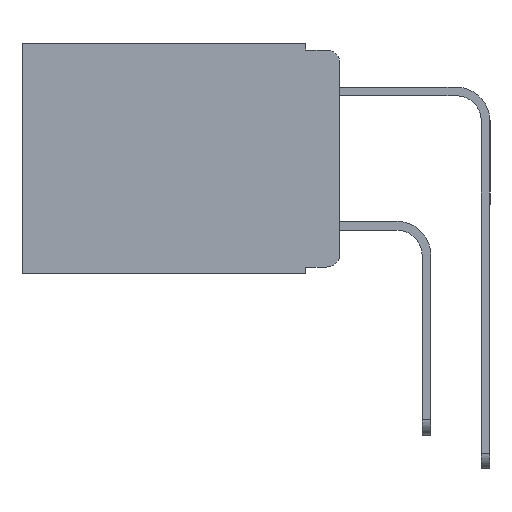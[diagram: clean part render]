
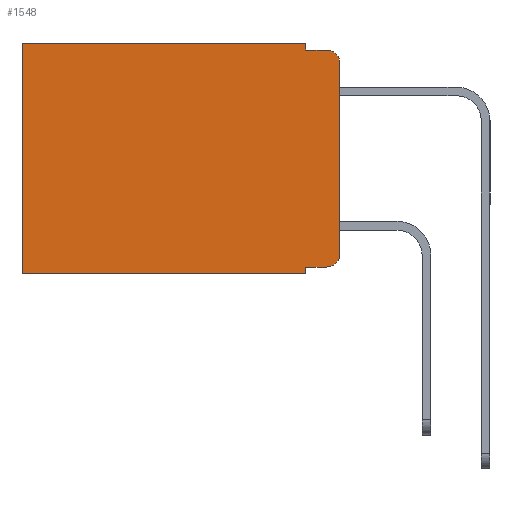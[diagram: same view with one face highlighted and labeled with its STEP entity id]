
A CAD part, left-side view. The second image highlights one B-rep face of the part: STEP entity #1548.
In plain terms, the highlighted planar face has unit normal (-1, 0, 0).
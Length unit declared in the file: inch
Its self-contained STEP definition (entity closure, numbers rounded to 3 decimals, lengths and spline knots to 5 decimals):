
#52 = VERTEX_POINT ( 'NONE', #1079 ) ;
#53 = CARTESIAN_POINT ( 'NONE',  ( 0.298, 0., 0. ) ) ;
#161 = CARTESIAN_POINT ( 'NONE',  ( 0.298, 0.473, 0. ) ) ;
#314 = DIRECTION ( 'NONE',  ( -1., 0., 0. ) ) ;
#1079 = CARTESIAN_POINT ( 'NONE',  ( 0.298, 0.051, -0.333 ) ) ;
#1282 = VECTOR ( 'NONE', #4727, 39.37008 ) ;
#1391 = VERTEX_POINT ( 'NONE', #13516 ) ;
#1548 = ADVANCED_FACE ( 'NONE', ( #12957 ), #14495, .F. ) ;
#1565 = CARTESIAN_POINT ( 'NONE',  ( 0.298, 0., 0. ) ) ;
#1922 = LINE ( 'NONE', #53, #8721 ) ;
#2081 = AXIS2_PLACEMENT_3D ( 'NONE', #3588, #12886, #4955 ) ;
#2167 = AXIS2_PLACEMENT_3D ( 'NONE', #8548, #314, #9907 ) ;
#2639 = EDGE_LOOP ( 'NONE', ( #9447, #10034, #13676, #13838, #10603, #10833, #13771, #11213, #11817, #11562 ) ) ;
#2655 = DIRECTION ( 'NONE',  ( 0., 1., 0. ) ) ;
#2825 = VECTOR ( 'NONE', #10303, 39.37008 ) ;
#3288 = LINE ( 'NONE', #8969, #2825 ) ;
#3350 = CARTESIAN_POINT ( 'NONE',  ( 0.298, 0.051, 0. ) ) ;
#3588 = CARTESIAN_POINT ( 'NONE',  ( 0.298, 0.02, -0.313 ) ) ;
#3645 = DIRECTION ( 'NONE',  ( 0., 0., -1. ) ) ;
#3745 = VECTOR ( 'NONE', #2655, 39.37008 ) ;
#4056 = CARTESIAN_POINT ( 'NONE',  ( 0.298, 0.473, -0.343 ) ) ;
#4166 = CIRCLE ( 'NONE', #2081, 0.02 ) ;
#4727 = DIRECTION ( 'NONE',  ( 0., 0., -1. ) ) ;
#4955 = DIRECTION ( 'NONE',  ( 0., 0., -1. ) ) ;
#5181 = VECTOR ( 'NONE', #7122, 39.37008 ) ;
#5445 = LINE ( 'NONE', #9951, #8520 ) ;
#6330 = CARTESIAN_POINT ( 'NONE',  ( 0.298, 0.051, -0.343 ) ) ;
#6504 = LINE ( 'NONE', #14199, #13085 ) ;
#6538 = CARTESIAN_POINT ( 'NONE',  ( 0.298, 0.051, -0.01 ) ) ;
#6722 = VERTEX_POINT ( 'NONE', #8576 ) ;
#6908 = LINE ( 'NONE', #16805, #13487 ) ;
#7121 = CIRCLE ( 'NONE', #2167, 0.02 ) ;
#7122 = DIRECTION ( 'NONE',  ( 0., 1., 0. ) ) ;
#7329 = LINE ( 'NONE', #10708, #3745 ) ;
#7433 = AXIS2_PLACEMENT_3D ( 'NONE', #1565, #11981, #8709 ) ;
#7658 = DIRECTION ( 'NONE',  ( 0., -1., 0. ) ) ;
#8223 = DIRECTION ( 'NONE',  ( 0., 0., -1. ) ) ;
#8451 = EDGE_CURVE ( 'NONE', #1391, #9365, #1922, .T. ) ;
#8520 = VECTOR ( 'NONE', #11329, 39.37008 ) ;
#8548 = CARTESIAN_POINT ( 'NONE',  ( 0.298, 0.02, -0.03 ) ) ;
#8576 = CARTESIAN_POINT ( 'NONE',  ( 0.298, 0.051, 0. ) ) ;
#8709 = DIRECTION ( 'NONE',  ( 0., 0., -1. ) ) ;
#8721 = VECTOR ( 'NONE', #8223, 39.37008 ) ;
#8969 = CARTESIAN_POINT ( 'NONE',  ( 0.298, 0.051, 0. ) ) ;
#9130 = EDGE_CURVE ( 'NONE', #12515, #11247, #15687, .T. ) ;
#9365 = VERTEX_POINT ( 'NONE', #13101 ) ;
#9447 = ORIENTED_EDGE ( 'NONE', *, *, #8451, .F. ) ;
#9839 = EDGE_CURVE ( 'NONE', #6722, #12307, #7329, .T. ) ;
#9907 = DIRECTION ( 'NONE',  ( 0., 0., -1. ) ) ;
#9951 = CARTESIAN_POINT ( 'NONE',  ( 0.298, 0.051, -0.01 ) ) ;
#10033 = EDGE_CURVE ( 'NONE', #1391, #11646, #7121, .T. ) ;
#10034 = ORIENTED_EDGE ( 'NONE', *, *, #10033, .T. ) ;
#10087 = EDGE_CURVE ( 'NONE', #13814, #11646, #5445, .T. ) ;
#10092 = EDGE_CURVE ( 'NONE', #6722, #13814, #12052, .T. ) ;
#10171 = EDGE_CURVE ( 'NONE', #14672, #9365, #4166, .T. ) ;
#10187 = EDGE_CURVE ( 'NONE', #52, #14672, #6908, .T. ) ;
#10192 = EDGE_CURVE ( 'NONE', #52, #12515, #3288, .T. ) ;
#10194 = EDGE_CURVE ( 'NONE', #12307, #11247, #6504, .T. ) ;
#10303 = DIRECTION ( 'NONE',  ( 0., 0., -1. ) ) ;
#10603 = ORIENTED_EDGE ( 'NONE', *, *, #9839, .T. ) ;
#10708 = CARTESIAN_POINT ( 'NONE',  ( 0.298, 0., 0. ) ) ;
#10833 = ORIENTED_EDGE ( 'NONE', *, *, #10194, .T. ) ;
#11014 = CARTESIAN_POINT ( 'NONE',  ( 0.298, 0., -0.343 ) ) ;
#11213 = ORIENTED_EDGE ( 'NONE', *, *, #10192, .F. ) ;
#11247 = VERTEX_POINT ( 'NONE', #4056 ) ;
#11329 = DIRECTION ( 'NONE',  ( 0., -1., 0. ) ) ;
#11562 = ORIENTED_EDGE ( 'NONE', *, *, #10171, .T. ) ;
#11646 = VERTEX_POINT ( 'NONE', #12961 ) ;
#11817 = ORIENTED_EDGE ( 'NONE', *, *, #10187, .T. ) ;
#11981 = DIRECTION ( 'NONE',  ( 1., 0., 0. ) ) ;
#12052 = LINE ( 'NONE', #3350, #1282 ) ;
#12307 = VERTEX_POINT ( 'NONE', #161 ) ;
#12515 = VERTEX_POINT ( 'NONE', #6330 ) ;
#12886 = DIRECTION ( 'NONE',  ( -1., 0., 0. ) ) ;
#12957 = FACE_OUTER_BOUND ( 'NONE', #2639, .T. ) ;
#12961 = CARTESIAN_POINT ( 'NONE',  ( 0.298, 0.02, -0.01 ) ) ;
#13085 = VECTOR ( 'NONE', #3645, 39.37008 ) ;
#13101 = CARTESIAN_POINT ( 'NONE',  ( 0.298, 0., -0.313 ) ) ;
#13487 = VECTOR ( 'NONE', #7658, 39.37008 ) ;
#13516 = CARTESIAN_POINT ( 'NONE',  ( 0.298, 0., -0.03 ) ) ;
#13676 = ORIENTED_EDGE ( 'NONE', *, *, #10087, .F. ) ;
#13771 = ORIENTED_EDGE ( 'NONE', *, *, #9130, .F. ) ;
#13814 = VERTEX_POINT ( 'NONE', #6538 ) ;
#13838 = ORIENTED_EDGE ( 'NONE', *, *, #10092, .F. ) ;
#14199 = CARTESIAN_POINT ( 'NONE',  ( 0.298, 0.473, 0. ) ) ;
#14495 = PLANE ( 'NONE',  #7433 ) ;
#14672 = VERTEX_POINT ( 'NONE', #15317 ) ;
#15317 = CARTESIAN_POINT ( 'NONE',  ( 0.298, 0.02, -0.333 ) ) ;
#15687 = LINE ( 'NONE', #11014, #5181 ) ;
#16805 = CARTESIAN_POINT ( 'NONE',  ( 0.298, 0.051, -0.333 ) ) ;
